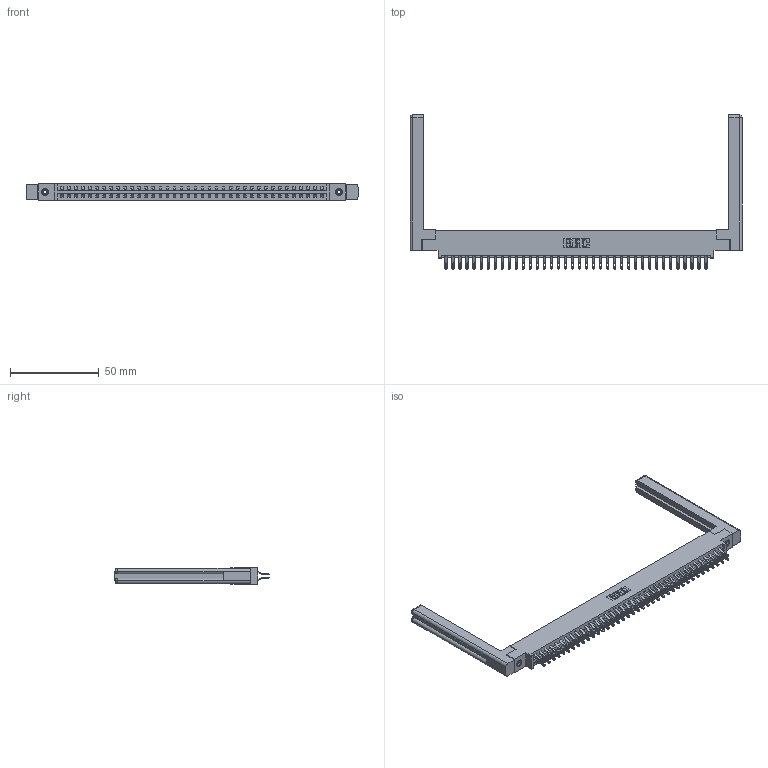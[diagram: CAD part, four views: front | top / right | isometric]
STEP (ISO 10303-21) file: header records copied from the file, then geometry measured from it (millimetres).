
FILE_DESCRIPTION (( 'STEP AP203' ), '1' );
FILE_NAME ('387-076-555-858.STEP', '2019-10-22T04:20:33', ( '' ), ( '' ), 'SwSTEP 2.0', 'SolidWorks 2016', '' );
FILE_SCHEMA (( 'CONFIG_CONTROL_DESIGN' ));
Length unit declared in the file: inch
Products named in the file (5): 387-076-555-858; 337 Part_0.170 Offset - 0.156 Dia-TI; 345-292-001_555 Tail; 345-250-001_345-250-001-102; 307-220-058
Assembly tree (81 placements, depth 2):
  387-076-555-858
    337 Part_0.170 Offset - 0.156 Dia-TI
    345-292-001_555 Tail  x76
    345-250-001_345-250-001-102  x2
    307-220-058  x2
Bounding box: 187.2 x 86.87 x 9.4 mm (x, y, z)
Volume: 26920.4 mm3; surface area: 28305.7 mm2
Topology: 81 solids, 81 shells, 4820 faces, 15041 edges, 10014 vertices
Faces by surface type: plane 2894, cylinder 1902, cone 12, torus 12
Entity records: 33072 total; most frequent: CARTESIAN_POINT 5619, ORIENTED_EDGE 5464, DIRECTION 4772, EDGE_CURVE 2732, LINE 2536, VECTOR 2536, VERTEX_POINT 1814, AXIS2_PLACEMENT_3D 1118
